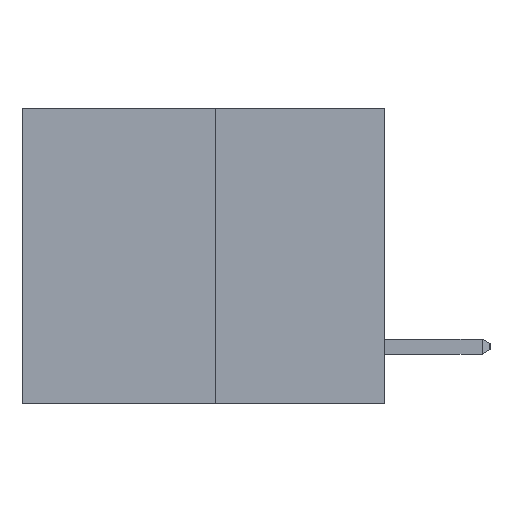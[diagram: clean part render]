
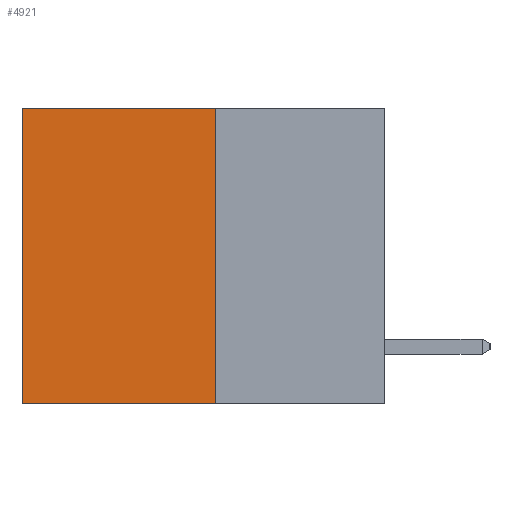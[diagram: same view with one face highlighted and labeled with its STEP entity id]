
A CAD part, left-side view. The second image highlights one B-rep face of the part: STEP entity #4921.
In plain terms, the highlighted planar face has unit normal (-1, 0, 0).
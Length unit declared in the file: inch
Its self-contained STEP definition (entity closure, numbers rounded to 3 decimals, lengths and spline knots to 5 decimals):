
#45 = VERTEX_POINT ( 'NONE', #21969 ) ;
#725 = EDGE_CURVE ( 'NONE', #45, #2336, #12216, .T. ) ;
#1494 = VECTOR ( 'NONE', #11640, 39.37008 ) ;
#2336 = VERTEX_POINT ( 'NONE', #13577 ) ;
#2383 = CARTESIAN_POINT ( 'NONE',  ( 0.3165, 0.28, -0.49 ) ) ;
#2417 = DIRECTION ( 'NONE',  ( 0., 0., -1. ) ) ;
#2604 = LINE ( 'NONE', #9065, #3112 ) ;
#3112 = VECTOR ( 'NONE', #8992, 39.37008 ) ;
#3585 = EDGE_CURVE ( 'NONE', #16219, #22278, #17452, .T. ) ;
#3866 = CARTESIAN_POINT ( 'NONE',  ( 0.3165, 0.28, 0. ) ) ;
#4116 = VECTOR ( 'NONE', #2417, 39.37008 ) ;
#4921 = ADVANCED_FACE ( 'NONE', ( #9627 ), #14208, .F. ) ;
#5615 = CARTESIAN_POINT ( 'NONE',  ( 0.3165, 0.28, -0.49 ) ) ;
#5645 = AXIS2_PLACEMENT_3D ( 'NONE', #5615, #17849, #17685 ) ;
#7096 = EDGE_CURVE ( 'NONE', #22278, #2336, #12811, .T. ) ;
#7174 = ORIENTED_EDGE ( 'NONE', *, *, #725, .T. ) ;
#8992 = DIRECTION ( 'NONE',  ( 0., 1., 0. ) ) ;
#9065 = CARTESIAN_POINT ( 'NONE',  ( 0.3165, 0.28, 0. ) ) ;
#9627 = FACE_OUTER_BOUND ( 'NONE', #21885, .T. ) ;
#10406 = CARTESIAN_POINT ( 'NONE',  ( 0.3165, 0.28, -0.49 ) ) ;
#11640 = DIRECTION ( 'NONE',  ( 0., 0., -1. ) ) ;
#11866 = ORIENTED_EDGE ( 'NONE', *, *, #14741, .T. ) ;
#12216 = LINE ( 'NONE', #16234, #4116 ) ;
#12811 = LINE ( 'NONE', #2383, #18207 ) ;
#13577 = CARTESIAN_POINT ( 'NONE',  ( 0.3165, 0.6, -0.49 ) ) ;
#14208 = PLANE ( 'NONE',  #5645 ) ;
#14741 = EDGE_CURVE ( 'NONE', #16219, #45, #2604, .T. ) ;
#15881 = ORIENTED_EDGE ( 'NONE', *, *, #7096, .F. ) ;
#16208 = DIRECTION ( 'NONE',  ( 0., 1., 0. ) ) ;
#16219 = VERTEX_POINT ( 'NONE', #3866 ) ;
#16234 = CARTESIAN_POINT ( 'NONE',  ( 0.3165, 0.6, -0.49 ) ) ;
#17452 = LINE ( 'NONE', #21959, #1494 ) ;
#17685 = DIRECTION ( 'NONE',  ( 0., 0., -1. ) ) ;
#17849 = DIRECTION ( 'NONE',  ( 1., 0., 0. ) ) ;
#18207 = VECTOR ( 'NONE', #16208, 39.37008 ) ;
#19675 = ORIENTED_EDGE ( 'NONE', *, *, #3585, .F. ) ;
#21885 = EDGE_LOOP ( 'NONE', ( #7174, #15881, #19675, #11866 ) ) ;
#21959 = CARTESIAN_POINT ( 'NONE',  ( 0.3165, 0.28, -0.49 ) ) ;
#21969 = CARTESIAN_POINT ( 'NONE',  ( 0.3165, 0.6, 0. ) ) ;
#22278 = VERTEX_POINT ( 'NONE', #10406 ) ;
